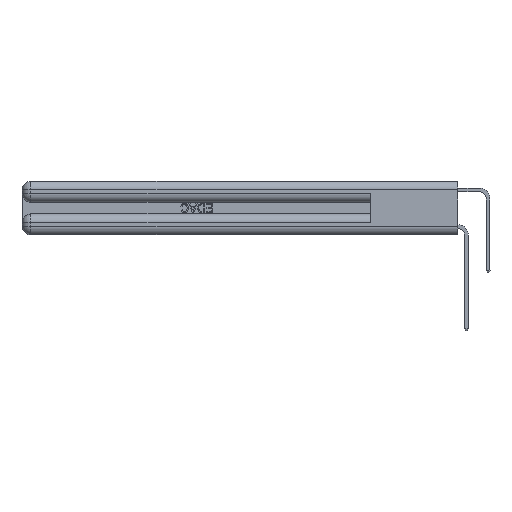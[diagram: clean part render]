
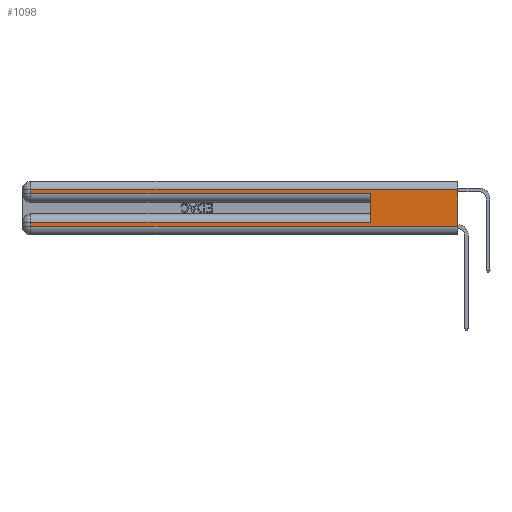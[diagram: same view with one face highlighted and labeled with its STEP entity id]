
A CAD part, left-side view. The second image highlights one B-rep face of the part: STEP entity #1098.
In plain terms, the highlighted planar face has unit normal (-1, 0, 0).
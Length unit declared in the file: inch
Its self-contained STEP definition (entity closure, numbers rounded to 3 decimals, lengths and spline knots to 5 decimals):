
#75 = DIRECTION ( 'NONE',  ( 0., -1., 0. ) ) ;
#1098 = ADVANCED_FACE ( 'NONE', ( #21006 ), #34632, .F. ) ;
#1245 = ORIENTED_EDGE ( 'NONE', *, *, #7301, .F. ) ;
#1781 = EDGE_CURVE ( 'NONE', #23266, #12220, #28363, .T. ) ;
#1936 = CARTESIAN_POINT ( 'NONE',  ( 0., 0., 0.37 ) ) ;
#1998 = CARTESIAN_POINT ( 'NONE',  ( 0., 2.94, 0.37 ) ) ;
#2134 = CARTESIAN_POINT ( 'NONE',  ( 0., 2.94, 0.06 ) ) ;
#3311 = DIRECTION ( 'NONE',  ( 0., 1., 0. ) ) ;
#4263 = VERTEX_POINT ( 'NONE', #30638 ) ;
#4352 = LINE ( 'NONE', #1998, #11049 ) ;
#5042 = LINE ( 'NONE', #16112, #12138 ) ;
#5501 = CARTESIAN_POINT ( 'NONE',  ( 0., 0.6, 0.145 ) ) ;
#5556 = VERTEX_POINT ( 'NONE', #11263 ) ;
#6702 = LINE ( 'NONE', #17941, #18941 ) ;
#7301 = EDGE_CURVE ( 'NONE', #23266, #4263, #21480, .T. ) ;
#7597 = DIRECTION ( 'NONE',  ( 1., 0., 0. ) ) ;
#7650 = VERTEX_POINT ( 'NONE', #23786 ) ;
#7922 = ORIENTED_EDGE ( 'NONE', *, *, #31405, .T. ) ;
#8253 = DIRECTION ( 'NONE',  ( 0., 0., 1. ) ) ;
#8455 = CARTESIAN_POINT ( 'NONE',  ( 0., 0., 0.085 ) ) ;
#8856 = VECTOR ( 'NONE', #8253, 39.37008 ) ;
#9890 = CARTESIAN_POINT ( 'NONE',  ( 0., 0., 0.37 ) ) ;
#9905 = VERTEX_POINT ( 'NONE', #18441 ) ;
#11049 = VECTOR ( 'NONE', #23597, 39.37008 ) ;
#11195 = ORIENTED_EDGE ( 'NONE', *, *, #26806, .T. ) ;
#11263 = CARTESIAN_POINT ( 'NONE',  ( 0., 2.94, 0.31 ) ) ;
#11889 = EDGE_CURVE ( 'NONE', #33378, #7650, #23020, .T. ) ;
#11895 = DIRECTION ( 'NONE',  ( 0., 0., -1. ) ) ;
#12138 = VECTOR ( 'NONE', #27167, 39.37008 ) ;
#12220 = VERTEX_POINT ( 'NONE', #27901 ) ;
#12288 = ORIENTED_EDGE ( 'NONE', *, *, #21725, .F. ) ;
#12432 = LINE ( 'NONE', #9890, #23343 ) ;
#12505 = DIRECTION ( 'NONE',  ( 0., 0., -1. ) ) ;
#12812 = EDGE_LOOP ( 'NONE', ( #12288, #30165, #7922, #24813, #1245, #19113, #11195, #15403 ) ) ;
#15403 = ORIENTED_EDGE ( 'NONE', *, *, #11889, .T. ) ;
#15667 = EDGE_CURVE ( 'NONE', #9905, #5556, #5042, .T. ) ;
#15694 = VERTEX_POINT ( 'NONE', #28024 ) ;
#16112 = CARTESIAN_POINT ( 'NONE',  ( 0., 0., 0.31 ) ) ;
#16664 = VECTOR ( 'NONE', #28653, 39.37008 ) ;
#17941 = CARTESIAN_POINT ( 'NONE',  ( 0., 2.94, 0.37 ) ) ;
#18441 = CARTESIAN_POINT ( 'NONE',  ( 0., 0., 0.31 ) ) ;
#18941 = VECTOR ( 'NONE', #12505, 39.37008 ) ;
#19113 = ORIENTED_EDGE ( 'NONE', *, *, #1781, .T. ) ;
#20652 = DIRECTION ( 'NONE',  ( 0., 0., -1. ) ) ;
#21006 = FACE_OUTER_BOUND ( 'NONE', #12812, .T. ) ;
#21480 = LINE ( 'NONE', #5501, #8856 ) ;
#21725 = EDGE_CURVE ( 'NONE', #9905, #7650, #12432, .T. ) ;
#22265 = AXIS2_PLACEMENT_3D ( 'NONE', #1936, #7597, #20652 ) ;
#23020 = LINE ( 'NONE', #29013, #16664 ) ;
#23266 = VERTEX_POINT ( 'NONE', #32376 ) ;
#23343 = VECTOR ( 'NONE', #11895, 39.37008 ) ;
#23597 = DIRECTION ( 'NONE',  ( 0., 0., -1. ) ) ;
#23786 = CARTESIAN_POINT ( 'NONE',  ( 0., 0., 0.06 ) ) ;
#24567 = EDGE_CURVE ( 'NONE', #15694, #4263, #35488, .T. ) ;
#24813 = ORIENTED_EDGE ( 'NONE', *, *, #24567, .T. ) ;
#24920 = CARTESIAN_POINT ( 'NONE',  ( 0., 0., 0.285 ) ) ;
#26806 = EDGE_CURVE ( 'NONE', #12220, #33378, #6702, .T. ) ;
#27167 = DIRECTION ( 'NONE',  ( 0., 1., 0. ) ) ;
#27327 = VECTOR ( 'NONE', #3311, 39.37008 ) ;
#27901 = CARTESIAN_POINT ( 'NONE',  ( 0., 2.94, 0.085 ) ) ;
#28024 = CARTESIAN_POINT ( 'NONE',  ( 0., 2.94, 0.285 ) ) ;
#28363 = LINE ( 'NONE', #8455, #27327 ) ;
#28653 = DIRECTION ( 'NONE',  ( 0., -1., 0. ) ) ;
#29013 = CARTESIAN_POINT ( 'NONE',  ( 0., 0., 0.06 ) ) ;
#30165 = ORIENTED_EDGE ( 'NONE', *, *, #15667, .T. ) ;
#30638 = CARTESIAN_POINT ( 'NONE',  ( 0., 0.6, 0.285 ) ) ;
#31073 = VECTOR ( 'NONE', #75, 39.37008 ) ;
#31405 = EDGE_CURVE ( 'NONE', #5556, #15694, #4352, .T. ) ;
#32376 = CARTESIAN_POINT ( 'NONE',  ( 0., 0.6, 0.085 ) ) ;
#33378 = VERTEX_POINT ( 'NONE', #2134 ) ;
#34632 = PLANE ( 'NONE',  #22265 ) ;
#35488 = LINE ( 'NONE', #24920, #31073 ) ;
